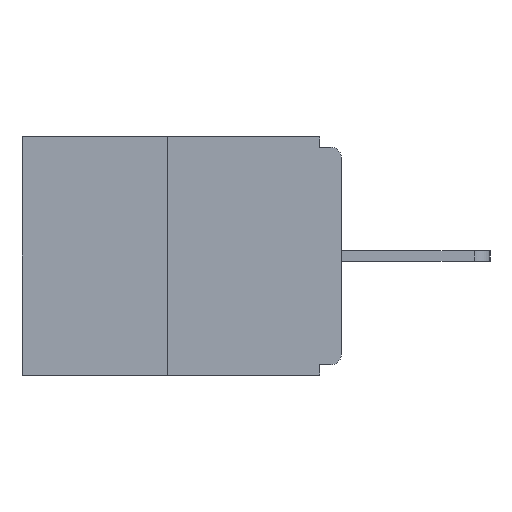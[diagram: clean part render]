
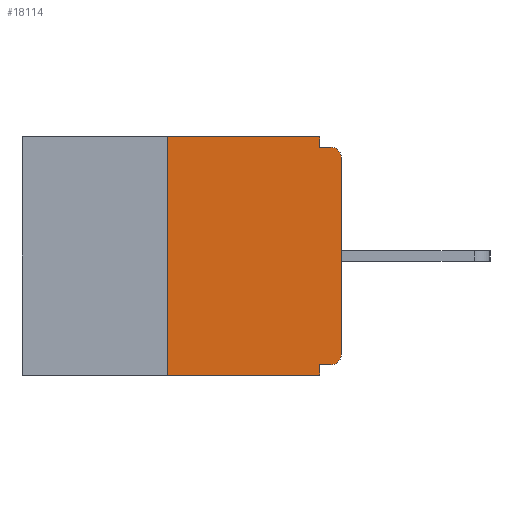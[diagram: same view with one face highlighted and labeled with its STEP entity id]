
A CAD part, left-side view. The second image highlights one B-rep face of the part: STEP entity #18114.
In plain terms, the highlighted planar face has unit normal (-1, 0, 0).
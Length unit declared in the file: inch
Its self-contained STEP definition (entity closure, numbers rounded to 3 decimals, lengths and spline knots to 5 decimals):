
#502 = CARTESIAN_POINT ( 'NONE',  ( 0., 0.015, -0.03 ) ) ;
#951 = VECTOR ( 'NONE', #26007, 39.37008 ) ;
#1231 = DIRECTION ( 'NONE',  ( 0., -1., 0. ) ) ;
#1750 = EDGE_CURVE ( 'NONE', #7215, #14789, #17312, .T. ) ;
#2694 = LINE ( 'NONE', #15080, #5458 ) ;
#3189 = ORIENTED_EDGE ( 'NONE', *, *, #22517, .F. ) ;
#3217 = VERTEX_POINT ( 'NONE', #5245 ) ;
#3345 = VECTOR ( 'NONE', #1231, 39.37008 ) ;
#3365 = LINE ( 'NONE', #5359, #3345 ) ;
#4041 = VECTOR ( 'NONE', #15357, 39.37008 ) ;
#4362 = CARTESIAN_POINT ( 'NONE',  ( 0., 0.015, -0.313 ) ) ;
#4621 = CARTESIAN_POINT ( 'NONE',  ( 0., 0.46, 0. ) ) ;
#4735 = PLANE ( 'NONE',  #10450 ) ;
#5245 = CARTESIAN_POINT ( 'NONE',  ( 0., 0.031, 0. ) ) ;
#5359 = CARTESIAN_POINT ( 'NONE',  ( 0., 0.46, -0.343 ) ) ;
#5458 = VECTOR ( 'NONE', #16937, 39.37008 ) ;
#5682 = LINE ( 'NONE', #17922, #951 ) ;
#6215 = CIRCLE ( 'NONE', #11710, 0.015 ) ;
#6321 = VERTEX_POINT ( 'NONE', #20014 ) ;
#6861 = LINE ( 'NONE', #8734, #4041 ) ;
#6864 = DIRECTION ( 'NONE',  ( 0., 0., -1. ) ) ;
#7151 = EDGE_LOOP ( 'NONE', ( #24754, #21876, #8137, #3189, #12560, #14894, #13672, #15518, #16073, #21542 ) ) ;
#7211 = DIRECTION ( 'NONE',  ( 0., 0., 1. ) ) ;
#7215 = VERTEX_POINT ( 'NONE', #26023 ) ;
#7375 = EDGE_CURVE ( 'NONE', #21099, #7215, #24601, .T. ) ;
#7594 = CARTESIAN_POINT ( 'NONE',  ( 0., 0., -0.03 ) ) ;
#7818 = DIRECTION ( 'NONE',  ( 0., -1., 0. ) ) ;
#8137 = ORIENTED_EDGE ( 'NONE', *, *, #22690, .T. ) ;
#8734 = CARTESIAN_POINT ( 'NONE',  ( 0., 0., -0.015 ) ) ;
#8764 = CARTESIAN_POINT ( 'NONE',  ( 0., 0.015, -0.328 ) ) ;
#9809 = LINE ( 'NONE', #15649, #19934 ) ;
#9881 = LINE ( 'NONE', #24095, #11047 ) ;
#10450 = AXIS2_PLACEMENT_3D ( 'NONE', #4621, #12723, #6864 ) ;
#10722 = FACE_OUTER_BOUND ( 'NONE', #7151, .T. ) ;
#11047 = VECTOR ( 'NONE', #23345, 39.37008 ) ;
#11512 = CARTESIAN_POINT ( 'NONE',  ( 0., 0.031, -0.343 ) ) ;
#11710 = AXIS2_PLACEMENT_3D ( 'NONE', #502, #16590, #17095 ) ;
#11787 = VERTEX_POINT ( 'NONE', #18468 ) ;
#12405 = VECTOR ( 'NONE', #7211, 39.37008 ) ;
#12560 = ORIENTED_EDGE ( 'NONE', *, *, #24164, .F. ) ;
#12723 = DIRECTION ( 'NONE',  ( 1., 0., 0. ) ) ;
#13149 = AXIS2_PLACEMENT_3D ( 'NONE', #4362, #23087, #24809 ) ;
#13350 = VECTOR ( 'NONE', #15633, 39.37008 ) ;
#13376 = VERTEX_POINT ( 'NONE', #11512 ) ;
#13416 = EDGE_CURVE ( 'NONE', #24450, #3217, #9809, .T. ) ;
#13494 = LINE ( 'NONE', #21633, #13350 ) ;
#13672 = ORIENTED_EDGE ( 'NONE', *, *, #1750, .T. ) ;
#14789 = VERTEX_POINT ( 'NONE', #7594 ) ;
#14894 = ORIENTED_EDGE ( 'NONE', *, *, #7375, .T. ) ;
#15080 = CARTESIAN_POINT ( 'NONE',  ( 0., 0.031, -0.343 ) ) ;
#15357 = DIRECTION ( 'NONE',  ( 0., -1., 0. ) ) ;
#15467 = EDGE_CURVE ( 'NONE', #16517, #20809, #6861, .T. ) ;
#15518 = ORIENTED_EDGE ( 'NONE', *, *, #19372, .T. ) ;
#15521 = EDGE_CURVE ( 'NONE', #3217, #16517, #13494, .T. ) ;
#15633 = DIRECTION ( 'NONE',  ( 0., 0., -1. ) ) ;
#15649 = CARTESIAN_POINT ( 'NONE',  ( 0., 0.46, 0. ) ) ;
#15690 = CARTESIAN_POINT ( 'NONE',  ( 0., 0.015, -0.015 ) ) ;
#16073 = ORIENTED_EDGE ( 'NONE', *, *, #15467, .F. ) ;
#16517 = VERTEX_POINT ( 'NONE', #17721 ) ;
#16590 = DIRECTION ( 'NONE',  ( -1., 0., 0. ) ) ;
#16937 = DIRECTION ( 'NONE',  ( 0., 0., -1. ) ) ;
#17095 = DIRECTION ( 'NONE',  ( 0., 0., -1. ) ) ;
#17290 = CARTESIAN_POINT ( 'NONE',  ( 0., 0.25, 0. ) ) ;
#17312 = LINE ( 'NONE', #25415, #12405 ) ;
#17721 = CARTESIAN_POINT ( 'NONE',  ( 0., 0.031, -0.015 ) ) ;
#17922 = CARTESIAN_POINT ( 'NONE',  ( 0., 0.25, 0. ) ) ;
#18114 = ADVANCED_FACE ( 'NONE', ( #10722 ), #4735, .F. ) ;
#18468 = CARTESIAN_POINT ( 'NONE',  ( 0., 0.031, -0.328 ) ) ;
#19372 = EDGE_CURVE ( 'NONE', #14789, #20809, #6215, .T. ) ;
#19934 = VECTOR ( 'NONE', #7818, 39.37008 ) ;
#20014 = CARTESIAN_POINT ( 'NONE',  ( 0., 0.25, -0.343 ) ) ;
#20809 = VERTEX_POINT ( 'NONE', #15690 ) ;
#21099 = VERTEX_POINT ( 'NONE', #8764 ) ;
#21542 = ORIENTED_EDGE ( 'NONE', *, *, #15521, .F. ) ;
#21633 = CARTESIAN_POINT ( 'NONE',  ( 0., 0.031, 0. ) ) ;
#21876 = ORIENTED_EDGE ( 'NONE', *, *, #26227, .F. ) ;
#22517 = EDGE_CURVE ( 'NONE', #11787, #13376, #2694, .T. ) ;
#22690 = EDGE_CURVE ( 'NONE', #6321, #13376, #3365, .T. ) ;
#23087 = DIRECTION ( 'NONE',  ( -1., 0., 0. ) ) ;
#23345 = DIRECTION ( 'NONE',  ( 0., 1., 0. ) ) ;
#24095 = CARTESIAN_POINT ( 'NONE',  ( 0., 0., -0.328 ) ) ;
#24164 = EDGE_CURVE ( 'NONE', #21099, #11787, #9881, .T. ) ;
#24450 = VERTEX_POINT ( 'NONE', #17290 ) ;
#24601 = CIRCLE ( 'NONE', #13149, 0.015 ) ;
#24754 = ORIENTED_EDGE ( 'NONE', *, *, #13416, .F. ) ;
#24809 = DIRECTION ( 'NONE',  ( 0., 0., -1. ) ) ;
#25415 = CARTESIAN_POINT ( 'NONE',  ( 0., 0., 0. ) ) ;
#26007 = DIRECTION ( 'NONE',  ( 0., 0., 1. ) ) ;
#26023 = CARTESIAN_POINT ( 'NONE',  ( 0., 0., -0.313 ) ) ;
#26227 = EDGE_CURVE ( 'NONE', #6321, #24450, #5682, .T. ) ;
